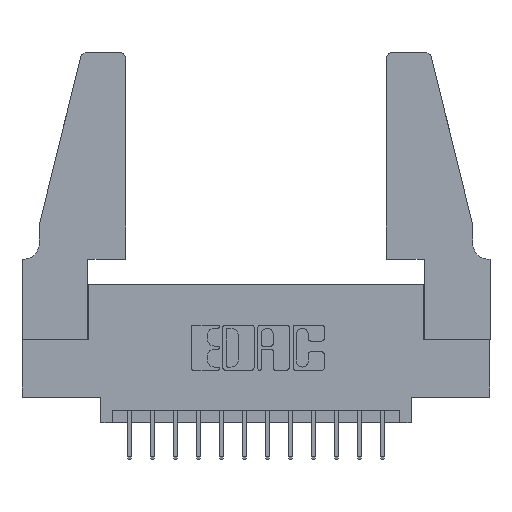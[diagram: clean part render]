
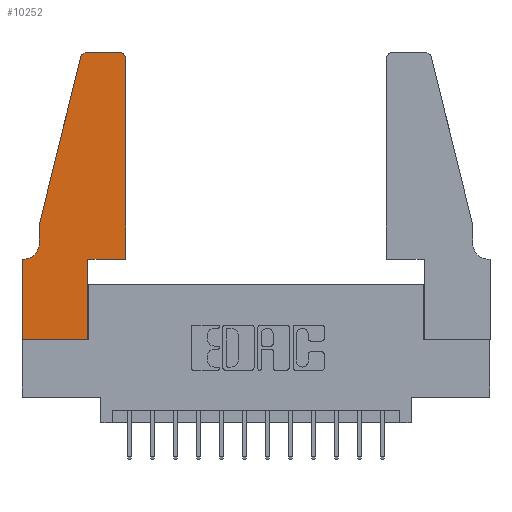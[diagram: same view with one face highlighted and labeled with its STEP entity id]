
A CAD part, top view. The second image highlights one B-rep face of the part: STEP entity #10252.
In plain terms, the highlighted planar face has unit normal (0, 0, 1).
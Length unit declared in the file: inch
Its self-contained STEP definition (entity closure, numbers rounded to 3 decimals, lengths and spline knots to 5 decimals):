
#148 = CARTESIAN_POINT ( 'NONE',  ( 0.0755, 0.42, 0.37 ) ) ;
#248 = CARTESIAN_POINT ( 'NONE',  ( 0.2865, 0.35, 0.37 ) ) ;
#293 = EDGE_CURVE ( 'NONE', #10248, #6601, #3751, .T. ) ;
#412 = EDGE_CURVE ( 'NONE', #6497, #1454, #4691, .T. ) ;
#615 = ORIENTED_EDGE ( 'NONE', *, *, #4722, .T. ) ;
#628 = EDGE_CURVE ( 'NONE', #7419, #14514, #7893, .T. ) ;
#671 = CIRCLE ( 'NONE', #7077, 0.03 ) ;
#806 = DIRECTION ( 'NONE',  ( -1., 0., 0. ) ) ;
#1079 = DIRECTION ( 'NONE',  ( 1., 0., 0. ) ) ;
#1121 = DIRECTION ( 'NONE',  ( 0., 0., 1. ) ) ;
#1174 = CARTESIAN_POINT ( 'NONE',  ( 0.4505, 0.35, 0.37 ) ) ;
#1247 = VERTEX_POINT ( 'NONE', #4737 ) ;
#1372 = LINE ( 'NONE', #12736, #12033 ) ;
#1454 = VERTEX_POINT ( 'NONE', #12236 ) ;
#1496 = DIRECTION ( 'NONE',  ( 0., -1., 0. ) ) ;
#1757 = LINE ( 'NONE', #15584, #1946 ) ;
#1946 = VECTOR ( 'NONE', #806, 39.37008 ) ;
#1971 = DIRECTION ( 'NONE',  ( 0., 1., 0. ) ) ;
#2241 = CARTESIAN_POINT ( 'NONE',  ( 0., 0.35, 0.37 ) ) ;
#2242 = ORIENTED_EDGE ( 'NONE', *, *, #412, .T. ) ;
#2274 = AXIS2_PLACEMENT_3D ( 'NONE', #15077, #10040, #8685 ) ;
#2311 = EDGE_CURVE ( 'NONE', #9934, #1247, #9388, .T. ) ;
#2345 = ORIENTED_EDGE ( 'NONE', *, *, #2311, .T. ) ;
#2432 = VERTEX_POINT ( 'NONE', #13372 ) ;
#2475 = VERTEX_POINT ( 'NONE', #7637 ) ;
#2930 = CARTESIAN_POINT ( 'NONE',  ( 0.0755, 0.5, 0.37 ) ) ;
#3107 = ORIENTED_EDGE ( 'NONE', *, *, #293, .T. ) ;
#3335 = CARTESIAN_POINT ( 'NONE',  ( 0.0055, 0.42, 0.37 ) ) ;
#3734 = ORIENTED_EDGE ( 'NONE', *, *, #10182, .T. ) ;
#3741 = VECTOR ( 'NONE', #5227, 39.37008 ) ;
#3751 = LINE ( 'NONE', #248, #7909 ) ;
#3928 = CARTESIAN_POINT ( 'NONE',  ( 0., 0., 0.37 ) ) ;
#4116 = VERTEX_POINT ( 'NONE', #10759 ) ;
#4171 = EDGE_CURVE ( 'NONE', #6601, #2432, #15480, .T. ) ;
#4232 = CARTESIAN_POINT ( 'NONE',  ( 0.0755, 0.5, 0.37 ) ) ;
#4263 = CARTESIAN_POINT ( 'NONE',  ( 0.2865, 0.35, 0.37 ) ) ;
#4487 = EDGE_CURVE ( 'NONE', #1247, #4116, #12409, .T. ) ;
#4559 = EDGE_CURVE ( 'NONE', #4116, #10248, #1372, .T. ) ;
#4691 = CIRCLE ( 'NONE', #2274, 0.03 ) ;
#4722 = EDGE_CURVE ( 'NONE', #2432, #6497, #10868, .T. ) ;
#4737 = CARTESIAN_POINT ( 'NONE',  ( 0., 0.35, 0.37 ) ) ;
#4771 = VECTOR ( 'NONE', #1496, 39.37008 ) ;
#5227 = DIRECTION ( 'NONE',  ( -0.239, -0.971, 0. ) ) ;
#5465 = DIRECTION ( 'NONE',  ( 0., -1., 0. ) ) ;
#5560 = CARTESIAN_POINT ( 'NONE',  ( 0.4505, 1.22, 0.37 ) ) ;
#5871 = EDGE_CURVE ( 'NONE', #14514, #15106, #10056, .T. ) ;
#6478 = AXIS2_PLACEMENT_3D ( 'NONE', #2241, #1121, #10883 ) ;
#6497 = VERTEX_POINT ( 'NONE', #5560 ) ;
#6601 = VERTEX_POINT ( 'NONE', #4263 ) ;
#7077 = AXIS2_PLACEMENT_3D ( 'NONE', #13451, #15700, #1079 ) ;
#7419 = VERTEX_POINT ( 'NONE', #14225 ) ;
#7541 = EDGE_CURVE ( 'NONE', #15106, #9934, #13929, .T. ) ;
#7610 = CARTESIAN_POINT ( 'NONE',  ( 0.0755, 0.35, 0.37 ) ) ;
#7637 = CARTESIAN_POINT ( 'NONE',  ( 0.284, 1.25, 0.37 ) ) ;
#7893 = LINE ( 'NONE', #13833, #3741 ) ;
#7909 = VECTOR ( 'NONE', #14324, 39.37008 ) ;
#8179 = VECTOR ( 'NONE', #1971, 39.37008 ) ;
#8311 = DIRECTION ( 'NONE',  ( -1., 0., 0. ) ) ;
#8685 = DIRECTION ( 'NONE',  ( 1., 0., 0. ) ) ;
#9388 = LINE ( 'NONE', #7610, #11892 ) ;
#9533 = PLANE ( 'NONE',  #6478 ) ;
#9934 = VERTEX_POINT ( 'NONE', #10444 ) ;
#10040 = DIRECTION ( 'NONE',  ( 0., 0., 1. ) ) ;
#10056 = LINE ( 'NONE', #4232, #10834 ) ;
#10182 = EDGE_CURVE ( 'NONE', #2475, #7419, #671, .T. ) ;
#10248 = VERTEX_POINT ( 'NONE', #12050 ) ;
#10252 = ADVANCED_FACE ( 'NONE', ( #10775 ), #9533, .T. ) ;
#10444 = CARTESIAN_POINT ( 'NONE',  ( 0.0055, 0.35, 0.37 ) ) ;
#10680 = VECTOR ( 'NONE', #14663, 39.37008 ) ;
#10759 = CARTESIAN_POINT ( 'NONE',  ( 0., 0., 0.37 ) ) ;
#10775 = FACE_OUTER_BOUND ( 'NONE', #11073, .T. ) ;
#10834 = VECTOR ( 'NONE', #5465, 39.37008 ) ;
#10868 = LINE ( 'NONE', #14074, #8179 ) ;
#10883 = DIRECTION ( 'NONE',  ( 1., 0., 0. ) ) ;
#11073 = EDGE_LOOP ( 'NONE', ( #15652, #3734, #15136, #15515, #12865, #2345, #11347, #14038, #3107, #11799, #615, #2242 ) ) ;
#11347 = ORIENTED_EDGE ( 'NONE', *, *, #4487, .T. ) ;
#11799 = ORIENTED_EDGE ( 'NONE', *, *, #4171, .T. ) ;
#11892 = VECTOR ( 'NONE', #14999, 39.37008 ) ;
#12033 = VECTOR ( 'NONE', #13926, 39.37008 ) ;
#12050 = CARTESIAN_POINT ( 'NONE',  ( 0.2865, 0., 0.37 ) ) ;
#12236 = CARTESIAN_POINT ( 'NONE',  ( 0.4205, 1.25, 0.37 ) ) ;
#12409 = LINE ( 'NONE', #3928, #4771 ) ;
#12603 = EDGE_CURVE ( 'NONE', #1454, #2475, #1757, .T. ) ;
#12736 = CARTESIAN_POINT ( 'NONE',  ( 0., 0., 0.37 ) ) ;
#12865 = ORIENTED_EDGE ( 'NONE', *, *, #7541, .T. ) ;
#13098 = DIRECTION ( 'NONE',  ( 0., 0., -1. ) ) ;
#13372 = CARTESIAN_POINT ( 'NONE',  ( 0.4505, 0.35, 0.37 ) ) ;
#13430 = AXIS2_PLACEMENT_3D ( 'NONE', #3335, #13098, #8311 ) ;
#13451 = CARTESIAN_POINT ( 'NONE',  ( 0.284, 1.22, 0.37 ) ) ;
#13833 = CARTESIAN_POINT ( 'NONE',  ( 0.0755, 0.5, 0.37 ) ) ;
#13926 = DIRECTION ( 'NONE',  ( 1., 0., 0. ) ) ;
#13929 = CIRCLE ( 'NONE', #13430, 0.07 ) ;
#14038 = ORIENTED_EDGE ( 'NONE', *, *, #4559, .T. ) ;
#14074 = CARTESIAN_POINT ( 'NONE',  ( 0.4505, 0.35, 0.37 ) ) ;
#14225 = CARTESIAN_POINT ( 'NONE',  ( 0.25487, 1.22718, 0.37 ) ) ;
#14324 = DIRECTION ( 'NONE',  ( 0., 1., 0. ) ) ;
#14514 = VERTEX_POINT ( 'NONE', #2930 ) ;
#14663 = DIRECTION ( 'NONE',  ( 1., 0., 0. ) ) ;
#14999 = DIRECTION ( 'NONE',  ( -1., 0., 0. ) ) ;
#15077 = CARTESIAN_POINT ( 'NONE',  ( 0.4205, 1.22, 0.37 ) ) ;
#15106 = VERTEX_POINT ( 'NONE', #148 ) ;
#15136 = ORIENTED_EDGE ( 'NONE', *, *, #628, .T. ) ;
#15480 = LINE ( 'NONE', #1174, #10680 ) ;
#15515 = ORIENTED_EDGE ( 'NONE', *, *, #5871, .T. ) ;
#15584 = CARTESIAN_POINT ( 'NONE',  ( 0.2605, 1.25, 0.37 ) ) ;
#15652 = ORIENTED_EDGE ( 'NONE', *, *, #12603, .T. ) ;
#15700 = DIRECTION ( 'NONE',  ( 0., 0., 1. ) ) ;
